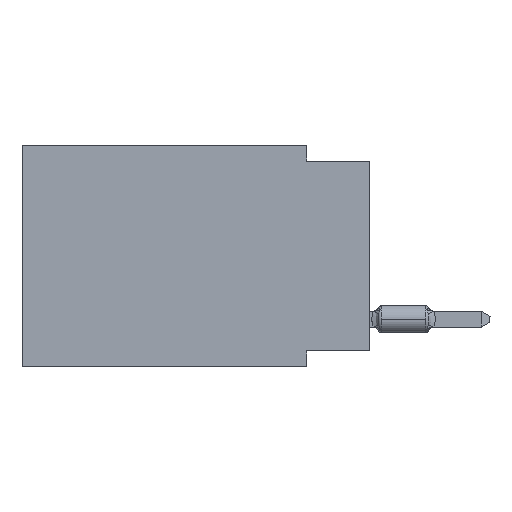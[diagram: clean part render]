
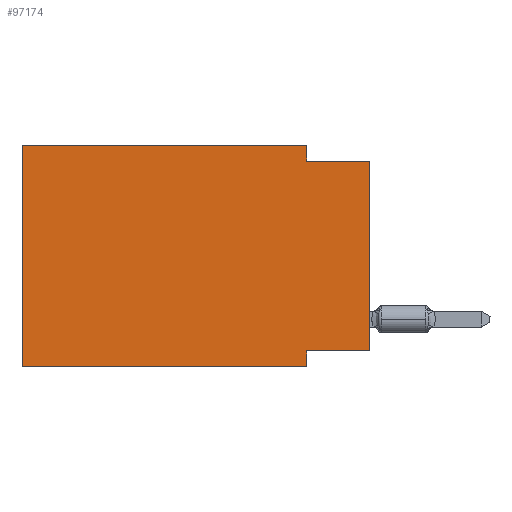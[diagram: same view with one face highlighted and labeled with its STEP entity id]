
A CAD part, left-side view. The second image highlights one B-rep face of the part: STEP entity #97174.
In plain terms, the highlighted planar face has unit normal (-1, 0, 0).
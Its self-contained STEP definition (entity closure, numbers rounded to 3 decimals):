
#598 = CARTESIAN_POINT ( 'NONE',  ( 0., 13.97, -8.89 ) ) ;
#992 = CARTESIAN_POINT ( 'NONE',  ( 0., 0., -8.255 ) ) ;
#3634 = EDGE_CURVE ( 'NONE', #82871, #90339, #95203, .T. ) ;
#5531 = DIRECTION ( 'NONE',  ( 0., 0., -1. ) ) ;
#8241 = EDGE_LOOP ( 'NONE', ( #78132, #38300, #96871, #82668, #86064, #56982, #97763, #8720 ) ) ;
#8720 = ORIENTED_EDGE ( 'NONE', *, *, #3634, .F. ) ;
#9056 = DIRECTION ( 'NONE',  ( 0., 0., 1. ) ) ;
#9323 = DIRECTION ( 'NONE',  ( 0., 1., 0. ) ) ;
#10236 = CARTESIAN_POINT ( 'NONE',  ( 0., 0., -0.635 ) ) ;
#10776 = EDGE_CURVE ( 'NONE', #29096, #53815, #76600, .T. ) ;
#13746 = EDGE_CURVE ( 'NONE', #33275, #29096, #15307, .T. ) ;
#13749 = CARTESIAN_POINT ( 'NONE',  ( 0., 2.54, -0.635 ) ) ;
#15307 = LINE ( 'NONE', #47559, #25693 ) ;
#15384 = LINE ( 'NONE', #48646, #63869 ) ;
#15903 = DIRECTION ( 'NONE',  ( 1., 0., 0. ) ) ;
#16158 = VERTEX_POINT ( 'NONE', #89904 ) ;
#16920 = VECTOR ( 'NONE', #47561, 1000. ) ;
#16983 = CARTESIAN_POINT ( 'NONE',  ( 0., 0., -8.255 ) ) ;
#17427 = DIRECTION ( 'NONE',  ( 0., -1., 0. ) ) ;
#22851 = EDGE_CURVE ( 'NONE', #90339, #16158, #55245, .T. ) ;
#25693 = VECTOR ( 'NONE', #45534, 1000. ) ;
#29096 = VERTEX_POINT ( 'NONE', #67376 ) ;
#30791 = CARTESIAN_POINT ( 'NONE',  ( 0., 2.54, -8.255 ) ) ;
#31764 = DIRECTION ( 'NONE',  ( 0., 0., 1. ) ) ;
#33275 = VERTEX_POINT ( 'NONE', #62845 ) ;
#34787 = DIRECTION ( 'NONE',  ( 0., -1., 0. ) ) ;
#38300 = ORIENTED_EDGE ( 'NONE', *, *, #39330, .F. ) ;
#39330 = EDGE_CURVE ( 'NONE', #53815, #72112, #86949, .T. ) ;
#42840 = EDGE_CURVE ( 'NONE', #91560, #33275, #15384, .T. ) ;
#42885 = EDGE_CURVE ( 'NONE', #91560, #16158, #49655, .T. ) ;
#43454 = AXIS2_PLACEMENT_3D ( 'NONE', #61957, #15903, #70621 ) ;
#45534 = DIRECTION ( 'NONE',  ( 0., -1., 0. ) ) ;
#47559 = CARTESIAN_POINT ( 'NONE',  ( 0., 13.97, 0. ) ) ;
#47561 = DIRECTION ( 'NONE',  ( 0., 0., -1. ) ) ;
#48646 = CARTESIAN_POINT ( 'NONE',  ( 0., 13.97, 0. ) ) ;
#49655 = LINE ( 'NONE', #81312, #80216 ) ;
#52229 = VECTOR ( 'NONE', #17427, 1000. ) ;
#53198 = CARTESIAN_POINT ( 'NONE',  ( 0., 0., -0.635 ) ) ;
#53815 = VERTEX_POINT ( 'NONE', #13749 ) ;
#54740 = CARTESIAN_POINT ( 'NONE',  ( 0., 2.54, -8.89 ) ) ;
#55245 = LINE ( 'NONE', #54740, #16920 ) ;
#55642 = CARTESIAN_POINT ( 'NONE',  ( 0., 0., 0. ) ) ;
#56982 = ORIENTED_EDGE ( 'NONE', *, *, #42885, .T. ) ;
#59946 = VECTOR ( 'NONE', #9323, 1000. ) ;
#61957 = CARTESIAN_POINT ( 'NONE',  ( 0., 13.97, 0. ) ) ;
#62845 = CARTESIAN_POINT ( 'NONE',  ( 0., 13.97, 0. ) ) ;
#63290 = LINE ( 'NONE', #55642, #74117 ) ;
#63869 = VECTOR ( 'NONE', #31764, 1000. ) ;
#67376 = CARTESIAN_POINT ( 'NONE',  ( 0., 2.54, 0. ) ) ;
#68803 = VECTOR ( 'NONE', #5531, 1000. ) ;
#68928 = CARTESIAN_POINT ( 'NONE',  ( 0., 2.54, 0. ) ) ;
#70621 = DIRECTION ( 'NONE',  ( 0., 0., -1. ) ) ;
#72112 = VERTEX_POINT ( 'NONE', #53198 ) ;
#74117 = VECTOR ( 'NONE', #9056, 1000. ) ;
#76600 = LINE ( 'NONE', #68928, #68803 ) ;
#78132 = ORIENTED_EDGE ( 'NONE', *, *, #83423, .T. ) ;
#80216 = VECTOR ( 'NONE', #34787, 1000. ) ;
#81312 = CARTESIAN_POINT ( 'NONE',  ( 0., 13.97, -8.89 ) ) ;
#82668 = ORIENTED_EDGE ( 'NONE', *, *, #13746, .F. ) ;
#82871 = VERTEX_POINT ( 'NONE', #992 ) ;
#83423 = EDGE_CURVE ( 'NONE', #82871, #72112, #63290, .T. ) ;
#85954 = PLANE ( 'NONE',  #43454 ) ;
#86064 = ORIENTED_EDGE ( 'NONE', *, *, #42840, .F. ) ;
#86949 = LINE ( 'NONE', #10236, #52229 ) ;
#89904 = CARTESIAN_POINT ( 'NONE',  ( 0., 2.54, -8.89 ) ) ;
#90339 = VERTEX_POINT ( 'NONE', #30791 ) ;
#91560 = VERTEX_POINT ( 'NONE', #598 ) ;
#95120 = FACE_OUTER_BOUND ( 'NONE', #8241, .T. ) ;
#95203 = LINE ( 'NONE', #16983, #59946 ) ;
#96871 = ORIENTED_EDGE ( 'NONE', *, *, #10776, .F. ) ;
#97174 = ADVANCED_FACE ( 'NONE', ( #95120 ), #85954, .F. ) ;
#97763 = ORIENTED_EDGE ( 'NONE', *, *, #22851, .F. ) ;
